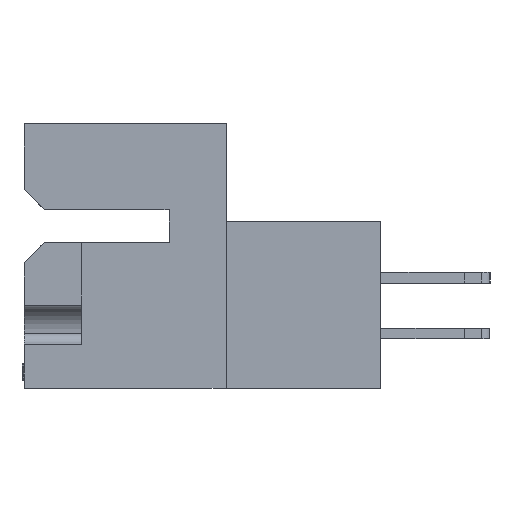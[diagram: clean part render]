
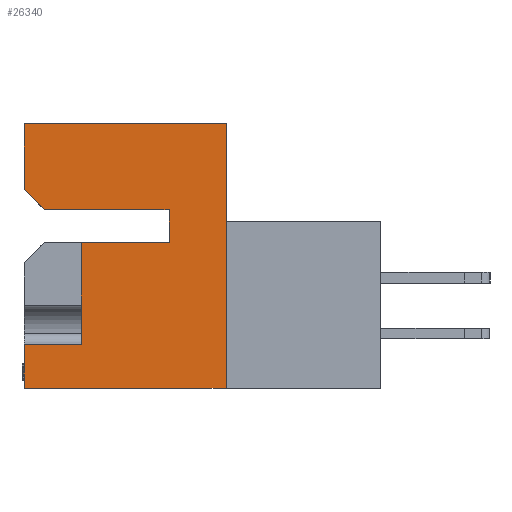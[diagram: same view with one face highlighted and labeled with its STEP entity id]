
A CAD part, left-side view. The second image highlights one B-rep face of the part: STEP entity #26340.
In plain terms, the highlighted planar face has unit normal (-1, 0, 0).
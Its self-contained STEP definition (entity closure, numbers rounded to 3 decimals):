
#100 = VECTOR ( 'NONE', #48861, 1000. ) ;
#1069 = AXIS2_PLACEMENT_3D ( 'NONE', #10039, #6371, #38003 ) ;
#1840 = ORIENTED_EDGE ( 'NONE', *, *, #32521, .F. ) ;
#2689 = EDGE_CURVE ( 'NONE', #11889, #29413, #7563, .T. ) ;
#3222 = LINE ( 'NONE', #20982, #100 ) ;
#3226 = CARTESIAN_POINT ( 'NONE',  ( 0., 11.506, 0. ) ) ;
#4479 = CARTESIAN_POINT ( 'NONE',  ( 0., -8.814, -15.088 ) ) ;
#4666 = VECTOR ( 'NONE', #6699, 1000. ) ;
#6061 = DIRECTION ( 'NONE',  ( 0., 0., 1. ) ) ;
#6371 = DIRECTION ( 'NONE',  ( 1., 0., 0. ) ) ;
#6699 = DIRECTION ( 'NONE',  ( 0., -1., 0. ) ) ;
#7563 = LINE ( 'NONE', #10412, #27563 ) ;
#9132 = EDGE_LOOP ( 'NONE', ( #11353, #25532, #21856, #33819, #31940, #13367, #15531, #26269, #1840, #17240, #29970 ) ) ;
#9362 = EDGE_CURVE ( 'NONE', #36402, #48232, #38899, .T. ) ;
#10039 = CARTESIAN_POINT ( 'NONE',  ( 0., 0., 0. ) ) ;
#10111 = LINE ( 'NONE', #31815, #25732 ) ;
#10135 = CARTESIAN_POINT ( 'NONE',  ( 0., 8.255, -12.58 ) ) ;
#10406 = VERTEX_POINT ( 'NONE', #46505 ) ;
#10412 = CARTESIAN_POINT ( 'NONE',  ( 0., 11.506, -15.088 ) ) ;
#10472 = LINE ( 'NONE', #39294, #26689 ) ;
#11353 = ORIENTED_EDGE ( 'NONE', *, *, #47604, .F. ) ;
#11889 = VERTEX_POINT ( 'NONE', #12400 ) ;
#12400 = CARTESIAN_POINT ( 'NONE',  ( 0., 11.506, -15.088 ) ) ;
#13035 = CARTESIAN_POINT ( 'NONE',  ( 0., 10.363, -4.902 ) ) ;
#13367 = ORIENTED_EDGE ( 'NONE', *, *, #9362, .F. ) ;
#14078 = CARTESIAN_POINT ( 'NONE',  ( 0., 0., -4.902 ) ) ;
#15531 = ORIENTED_EDGE ( 'NONE', *, *, #40340, .F. ) ;
#16829 = CARTESIAN_POINT ( 'NONE',  ( 0., 11.506, -3.759 ) ) ;
#17223 = VECTOR ( 'NONE', #32757, 1000. ) ;
#17240 = ORIENTED_EDGE ( 'NONE', *, *, #23566, .T. ) ;
#17350 = VERTEX_POINT ( 'NONE', #10135 ) ;
#17393 = EDGE_CURVE ( 'NONE', #27624, #48232, #10472, .T. ) ;
#18936 = VECTOR ( 'NONE', #48781, 1000. ) ;
#19820 = VECTOR ( 'NONE', #40768, 1000. ) ;
#19911 = FACE_OUTER_BOUND ( 'NONE', #9132, .T. ) ;
#20568 = CARTESIAN_POINT ( 'NONE',  ( 0., 3.251, -4.902 ) ) ;
#20982 = CARTESIAN_POINT ( 'NONE',  ( 0., 8.255, -6.782 ) ) ;
#21856 = ORIENTED_EDGE ( 'NONE', *, *, #28569, .F. ) ;
#22573 = CARTESIAN_POINT ( 'NONE',  ( 0., 0., -6.782 ) ) ;
#22891 = EDGE_CURVE ( 'NONE', #24469, #10406, #50833, .T. ) ;
#23566 = EDGE_CURVE ( 'NONE', #17350, #29413, #34197, .T. ) ;
#23829 = CARTESIAN_POINT ( 'NONE',  ( 0., 0., 0. ) ) ;
#24469 = VERTEX_POINT ( 'NONE', #31502 ) ;
#25079 = VERTEX_POINT ( 'NONE', #45504 ) ;
#25532 = ORIENTED_EDGE ( 'NONE', *, *, #22891, .F. ) ;
#25732 = VECTOR ( 'NONE', #47448, 1000. ) ;
#26269 = ORIENTED_EDGE ( 'NONE', *, *, #48614, .F. ) ;
#26286 = DIRECTION ( 'NONE',  ( 0., 1., 0. ) ) ;
#26340 = ADVANCED_FACE ( 'NONE', ( #19911 ), #49783, .F. ) ;
#26689 = VECTOR ( 'NONE', #43162, 1000. ) ;
#27563 = VECTOR ( 'NONE', #6061, 1000. ) ;
#27624 = VERTEX_POINT ( 'NONE', #16829 ) ;
#27798 = LINE ( 'NONE', #3226, #17223 ) ;
#28569 = EDGE_CURVE ( 'NONE', #25079, #24469, #27798, .T. ) ;
#29413 = VERTEX_POINT ( 'NONE', #29507 ) ;
#29507 = CARTESIAN_POINT ( 'NONE',  ( 0., 11.506, -12.58 ) ) ;
#29970 = ORIENTED_EDGE ( 'NONE', *, *, #2689, .F. ) ;
#30823 = CARTESIAN_POINT ( 'NONE',  ( 0., 11.506, -15.088 ) ) ;
#31502 = CARTESIAN_POINT ( 'NONE',  ( 0., 0., 0. ) ) ;
#31676 = EDGE_CURVE ( 'NONE', #27624, #25079, #32035, .T. ) ;
#31815 = CARTESIAN_POINT ( 'NONE',  ( 0., 3.251, -6.782 ) ) ;
#31940 = ORIENTED_EDGE ( 'NONE', *, *, #17393, .T. ) ;
#32035 = LINE ( 'NONE', #30823, #40868 ) ;
#32521 = EDGE_CURVE ( 'NONE', #17350, #50858, #3222, .T. ) ;
#32757 = DIRECTION ( 'NONE',  ( 0., -1., 0. ) ) ;
#33819 = ORIENTED_EDGE ( 'NONE', *, *, #31676, .F. ) ;
#34197 = LINE ( 'NONE', #44810, #19820 ) ;
#36402 = VERTEX_POINT ( 'NONE', #20568 ) ;
#38003 = DIRECTION ( 'NONE',  ( 0., 0., -1. ) ) ;
#38250 = VERTEX_POINT ( 'NONE', #48653 ) ;
#38899 = LINE ( 'NONE', #14078, #42684 ) ;
#39239 = DIRECTION ( 'NONE',  ( 0., 0., 1. ) ) ;
#39294 = CARTESIAN_POINT ( 'NONE',  ( 0., 10.363, -4.902 ) ) ;
#40125 = DIRECTION ( 'NONE',  ( 0., 0., -1. ) ) ;
#40235 = LINE ( 'NONE', #4479, #18936 ) ;
#40340 = EDGE_CURVE ( 'NONE', #38250, #36402, #10111, .T. ) ;
#40768 = DIRECTION ( 'NONE',  ( 0., 1., 0. ) ) ;
#40868 = VECTOR ( 'NONE', #39239, 1000. ) ;
#41023 = CARTESIAN_POINT ( 'NONE',  ( 0., 8.255, -6.782 ) ) ;
#42684 = VECTOR ( 'NONE', #26286, 1000. ) ;
#43162 = DIRECTION ( 'NONE',  ( 0., -0.707, -0.707 ) ) ;
#43262 = VECTOR ( 'NONE', #40125, 1000. ) ;
#44810 = CARTESIAN_POINT ( 'NONE',  ( 0., 8.255, -12.58 ) ) ;
#45504 = CARTESIAN_POINT ( 'NONE',  ( 0., 11.506, 0. ) ) ;
#46505 = CARTESIAN_POINT ( 'NONE',  ( 0., 0., -15.088 ) ) ;
#46617 = LINE ( 'NONE', #22573, #4666 ) ;
#47448 = DIRECTION ( 'NONE',  ( 0., 0., 1. ) ) ;
#47604 = EDGE_CURVE ( 'NONE', #10406, #11889, #40235, .T. ) ;
#48232 = VERTEX_POINT ( 'NONE', #13035 ) ;
#48614 = EDGE_CURVE ( 'NONE', #50858, #38250, #46617, .T. ) ;
#48653 = CARTESIAN_POINT ( 'NONE',  ( 0., 3.251, -6.782 ) ) ;
#48781 = DIRECTION ( 'NONE',  ( 0., 1., 0. ) ) ;
#48861 = DIRECTION ( 'NONE',  ( 0., 0., 1. ) ) ;
#49783 = PLANE ( 'NONE',  #1069 ) ;
#50833 = LINE ( 'NONE', #23829, #43262 ) ;
#50858 = VERTEX_POINT ( 'NONE', #41023 ) ;
